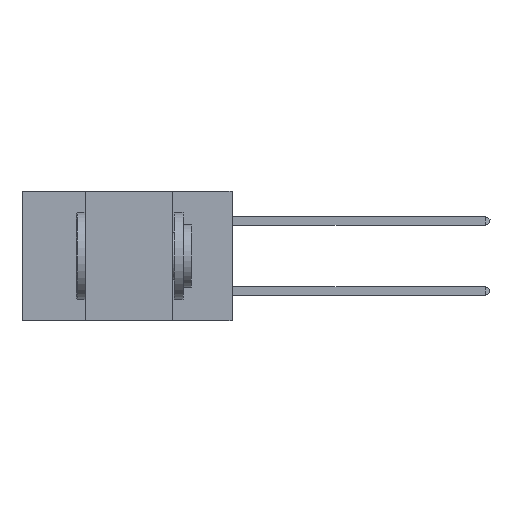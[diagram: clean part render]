
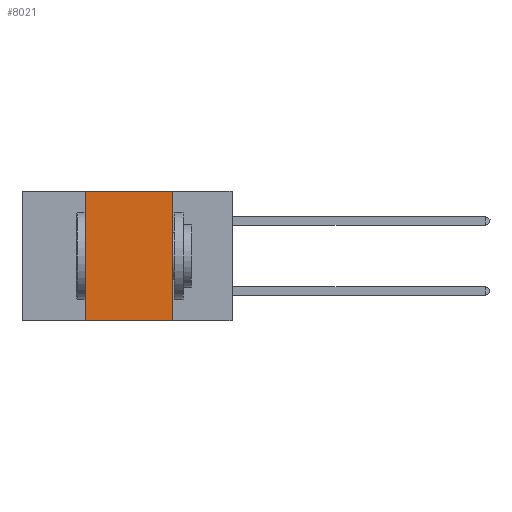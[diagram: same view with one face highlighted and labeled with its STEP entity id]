
A CAD part, left-side view. The second image highlights one B-rep face of the part: STEP entity #8021.
In plain terms, the highlighted planar face has unit normal (-1, 0, 0).
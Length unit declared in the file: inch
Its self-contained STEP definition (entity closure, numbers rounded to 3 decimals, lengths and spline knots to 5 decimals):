
#8 = DIRECTION ( 'NONE',  ( 0., -1., 0. ) ) ;
#909 = LINE ( 'NONE', #20165, #6048 ) ;
#1585 = ORIENTED_EDGE ( 'NONE', *, *, #18924, .F. ) ;
#1614 = ORIENTED_EDGE ( 'NONE', *, *, #8783, .F. ) ;
#1726 = DIRECTION ( 'NONE',  ( 0., 0., -1. ) ) ;
#2069 = EDGE_LOOP ( 'NONE', ( #1585, #1614, #12410, #17047 ) ) ;
#3296 = VECTOR ( 'NONE', #8, 39.37008 ) ;
#4968 = PLANE ( 'NONE',  #20847 ) ;
#5333 = LINE ( 'NONE', #14834, #3296 ) ;
#5545 = LINE ( 'NONE', #20564, #18334 ) ;
#5771 = CARTESIAN_POINT ( 'NONE',  ( 0., 0.6, 0. ) ) ;
#6048 = VECTOR ( 'NONE', #12130, 39.37008 ) ;
#6198 = LINE ( 'NONE', #5771, #18752 ) ;
#6680 = CARTESIAN_POINT ( 'NONE',  ( 0., 0.6, 0. ) ) ;
#7668 = DIRECTION ( 'NONE',  ( 0., -1., 0. ) ) ;
#8021 = ADVANCED_FACE ( 'NONE', ( #19537 ), #4968, .F. ) ;
#8598 = VERTEX_POINT ( 'NONE', #12740 ) ;
#8783 = EDGE_CURVE ( 'NONE', #17448, #11344, #6198, .T. ) ;
#9936 = DIRECTION ( 'NONE',  ( 1., 0., 0. ) ) ;
#10173 = CARTESIAN_POINT ( 'NONE',  ( 0., 0.17, -0.37 ) ) ;
#11344 = VERTEX_POINT ( 'NONE', #12524 ) ;
#12130 = DIRECTION ( 'NONE',  ( 0., 0., 1. ) ) ;
#12410 = ORIENTED_EDGE ( 'NONE', *, *, #19859, .F. ) ;
#12524 = CARTESIAN_POINT ( 'NONE',  ( 0., 0.17, 0. ) ) ;
#12740 = CARTESIAN_POINT ( 'NONE',  ( 0., 0.42, -0.37 ) ) ;
#12857 = VERTEX_POINT ( 'NONE', #10173 ) ;
#13476 = CARTESIAN_POINT ( 'NONE',  ( 0., 0.42, 0. ) ) ;
#14834 = CARTESIAN_POINT ( 'NONE',  ( 0., 0.6, -0.37 ) ) ;
#17047 = ORIENTED_EDGE ( 'NONE', *, *, #17950, .T. ) ;
#17397 = DIRECTION ( 'NONE',  ( 0., 0., -1. ) ) ;
#17448 = VERTEX_POINT ( 'NONE', #13476 ) ;
#17950 = EDGE_CURVE ( 'NONE', #8598, #12857, #5333, .T. ) ;
#18334 = VECTOR ( 'NONE', #17397, 39.37008 ) ;
#18752 = VECTOR ( 'NONE', #7668, 39.37008 ) ;
#18924 = EDGE_CURVE ( 'NONE', #11344, #12857, #5545, .T. ) ;
#19537 = FACE_OUTER_BOUND ( 'NONE', #2069, .T. ) ;
#19859 = EDGE_CURVE ( 'NONE', #8598, #17448, #909, .T. ) ;
#20165 = CARTESIAN_POINT ( 'NONE',  ( 0., 0.42, 0. ) ) ;
#20564 = CARTESIAN_POINT ( 'NONE',  ( 0., 0.17, 0. ) ) ;
#20847 = AXIS2_PLACEMENT_3D ( 'NONE', #6680, #9936, #1726 ) ;
